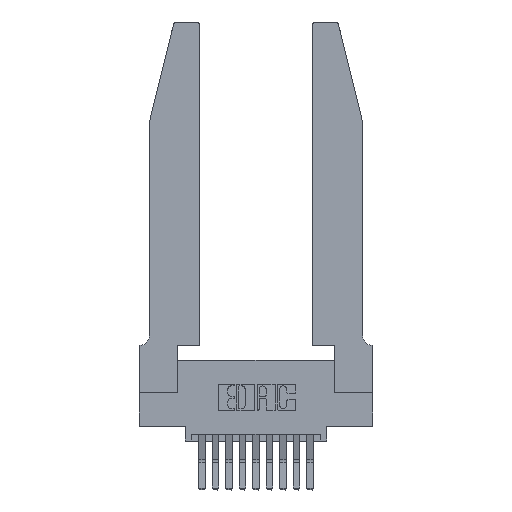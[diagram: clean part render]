
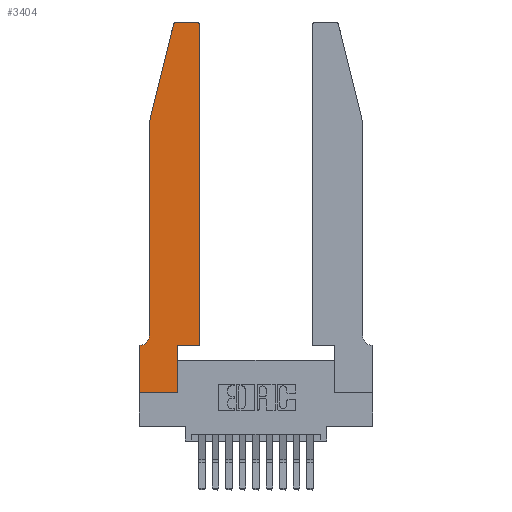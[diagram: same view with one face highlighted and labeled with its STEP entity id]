
A CAD part, top view. The second image highlights one B-rep face of the part: STEP entity #3404.
In plain terms, the highlighted planar face has unit normal (0, 0, 1).
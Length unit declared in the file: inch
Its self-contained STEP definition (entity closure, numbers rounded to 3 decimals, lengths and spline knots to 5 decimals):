
#18 = VERTEX_POINT ( 'NONE', #15408 ) ;
#112 = EDGE_CURVE ( 'NONE', #879, #8846, #6542, .T. ) ;
#124 = DIRECTION ( 'NONE',  ( -1., 0., 0. ) ) ;
#138 = EDGE_CURVE ( 'NONE', #18, #13343, #2961, .T. ) ;
#163 = CARTESIAN_POINT ( 'NONE',  ( 0.284, 2.75, 0.37 ) ) ;
#277 = ORIENTED_EDGE ( 'NONE', *, *, #13344, .T. ) ;
#594 = PLANE ( 'NONE',  #15920 ) ;
#720 = DIRECTION ( 'NONE',  ( 1., 0., 0. ) ) ;
#879 = VERTEX_POINT ( 'NONE', #12487 ) ;
#1127 = CARTESIAN_POINT ( 'NONE',  ( 0., 0., 0.37 ) ) ;
#1167 = VERTEX_POINT ( 'NONE', #163 ) ;
#1363 = CARTESIAN_POINT ( 'NONE',  ( 0.4205, 2.72, 0.37 ) ) ;
#1446 = EDGE_CURVE ( 'NONE', #7575, #16347, #2343, .T. ) ;
#1674 = EDGE_CURVE ( 'NONE', #16347, #2657, #2911, .T. ) ;
#1685 = VECTOR ( 'NONE', #15215, 39.37008 ) ;
#1941 = LINE ( 'NONE', #13389, #10059 ) ;
#2015 = EDGE_CURVE ( 'NONE', #1167, #12087, #8072, .T. ) ;
#2108 = LINE ( 'NONE', #13285, #8444 ) ;
#2284 = EDGE_CURVE ( 'NONE', #16276, #18, #13189, .T. ) ;
#2343 = LINE ( 'NONE', #15055, #3308 ) ;
#2656 = DIRECTION ( 'NONE',  ( 0., 0., 1. ) ) ;
#2657 = VERTEX_POINT ( 'NONE', #7000 ) ;
#2777 = DIRECTION ( 'NONE',  ( 1., 0., 0. ) ) ;
#2823 = FACE_OUTER_BOUND ( 'NONE', #12438, .T. ) ;
#2842 = EDGE_CURVE ( 'NONE', #13343, #1167, #3102, .T. ) ;
#2911 = CIRCLE ( 'NONE', #4374, 0.07 ) ;
#2961 = CIRCLE ( 'NONE', #4784, 0.03 ) ;
#3102 = LINE ( 'NONE', #14027, #4081 ) ;
#3308 = VECTOR ( 'NONE', #16214, 39.37008 ) ;
#3404 = ADVANCED_FACE ( 'NONE', ( #2823 ), #594, .T. ) ;
#4081 = VECTOR ( 'NONE', #6419, 39.37008 ) ;
#4095 = CARTESIAN_POINT ( 'NONE',  ( 0.284, 2.72, 0.37 ) ) ;
#4309 = DIRECTION ( 'NONE',  ( -0.239, -0.971, 0. ) ) ;
#4374 = AXIS2_PLACEMENT_3D ( 'NONE', #15332, #11326, #124 ) ;
#4407 = DIRECTION ( 'NONE',  ( 1., 0., 0. ) ) ;
#4457 = CARTESIAN_POINT ( 'NONE',  ( 0., 0.35, 0.37 ) ) ;
#4784 = AXIS2_PLACEMENT_3D ( 'NONE', #1363, #2656, #12595 ) ;
#5056 = CARTESIAN_POINT ( 'NONE',  ( 0.25487, 2.72718, 0.37 ) ) ;
#5128 = VECTOR ( 'NONE', #7625, 39.37008 ) ;
#5423 = VECTOR ( 'NONE', #2777, 39.37008 ) ;
#5799 = CARTESIAN_POINT ( 'NONE',  ( 0., 0.35, 0.37 ) ) ;
#5970 = EDGE_CURVE ( 'NONE', #2657, #6406, #1941, .T. ) ;
#6122 = ORIENTED_EDGE ( 'NONE', *, *, #2842, .T. ) ;
#6406 = VERTEX_POINT ( 'NONE', #5799 ) ;
#6419 = DIRECTION ( 'NONE',  ( -1., 0., 0. ) ) ;
#6542 = LINE ( 'NONE', #8840, #16332 ) ;
#7000 = CARTESIAN_POINT ( 'NONE',  ( 0.0055, 0.35, 0.37 ) ) ;
#7008 = VECTOR ( 'NONE', #720, 39.37008 ) ;
#7033 = DIRECTION ( 'NONE',  ( -1., 0., 0. ) ) ;
#7223 = EDGE_CURVE ( 'NONE', #12087, #7575, #2108, .T. ) ;
#7575 = VERTEX_POINT ( 'NONE', #13627 ) ;
#7625 = DIRECTION ( 'NONE',  ( 0., -1., 0. ) ) ;
#8072 = CIRCLE ( 'NONE', #9444, 0.03 ) ;
#8258 = VERTEX_POINT ( 'NONE', #1127 ) ;
#8377 = CARTESIAN_POINT ( 'NONE',  ( 0.4505, 0.35, 0.37 ) ) ;
#8444 = VECTOR ( 'NONE', #4309, 39.37008 ) ;
#8840 = CARTESIAN_POINT ( 'NONE',  ( 0.2865, 0.35, 0.37 ) ) ;
#8846 = VERTEX_POINT ( 'NONE', #12315 ) ;
#9150 = LINE ( 'NONE', #13397, #7008 ) ;
#9435 = ORIENTED_EDGE ( 'NONE', *, *, #7223, .T. ) ;
#9444 = AXIS2_PLACEMENT_3D ( 'NONE', #4095, #15449, #12951 ) ;
#10059 = VECTOR ( 'NONE', #7033, 39.37008 ) ;
#10223 = ORIENTED_EDGE ( 'NONE', *, *, #2015, .T. ) ;
#10348 = CARTESIAN_POINT ( 'NONE',  ( 0., 0., 0.37 ) ) ;
#10404 = EDGE_CURVE ( 'NONE', #8258, #879, #10953, .T. ) ;
#10598 = EDGE_CURVE ( 'NONE', #8846, #16276, #9150, .T. ) ;
#10953 = LINE ( 'NONE', #10348, #5423 ) ;
#11326 = DIRECTION ( 'NONE',  ( 0., 0., -1. ) ) ;
#11346 = CARTESIAN_POINT ( 'NONE',  ( 0.4505, 0.35, 0.37 ) ) ;
#11603 = CARTESIAN_POINT ( 'NONE',  ( 0.0755, 0.42, 0.37 ) ) ;
#12035 = LINE ( 'NONE', #15245, #5128 ) ;
#12087 = VERTEX_POINT ( 'NONE', #5056 ) ;
#12315 = CARTESIAN_POINT ( 'NONE',  ( 0.2865, 0.35, 0.37 ) ) ;
#12322 = ORIENTED_EDGE ( 'NONE', *, *, #10598, .T. ) ;
#12438 = EDGE_LOOP ( 'NONE', ( #6122, #10223, #9435, #13163, #14839, #13460, #277, #15935, #13560, #12322, #14319, #16209 ) ) ;
#12487 = CARTESIAN_POINT ( 'NONE',  ( 0.2865, 0., 0.37 ) ) ;
#12595 = DIRECTION ( 'NONE',  ( 1., 0., 0. ) ) ;
#12951 = DIRECTION ( 'NONE',  ( 1., 0., 0. ) ) ;
#13163 = ORIENTED_EDGE ( 'NONE', *, *, #1446, .T. ) ;
#13189 = LINE ( 'NONE', #8377, #1685 ) ;
#13285 = CARTESIAN_POINT ( 'NONE',  ( 0.0755, 2., 0.37 ) ) ;
#13343 = VERTEX_POINT ( 'NONE', #13937 ) ;
#13344 = EDGE_CURVE ( 'NONE', #6406, #8258, #12035, .T. ) ;
#13389 = CARTESIAN_POINT ( 'NONE',  ( 0.0755, 0.35, 0.37 ) ) ;
#13397 = CARTESIAN_POINT ( 'NONE',  ( 0.4505, 0.35, 0.37 ) ) ;
#13460 = ORIENTED_EDGE ( 'NONE', *, *, #5970, .T. ) ;
#13560 = ORIENTED_EDGE ( 'NONE', *, *, #112, .T. ) ;
#13627 = CARTESIAN_POINT ( 'NONE',  ( 0.0755, 2., 0.37 ) ) ;
#13937 = CARTESIAN_POINT ( 'NONE',  ( 0.4205, 2.75, 0.37 ) ) ;
#14027 = CARTESIAN_POINT ( 'NONE',  ( 0.2605, 2.75, 0.37 ) ) ;
#14319 = ORIENTED_EDGE ( 'NONE', *, *, #2284, .T. ) ;
#14839 = ORIENTED_EDGE ( 'NONE', *, *, #1674, .T. ) ;
#15055 = CARTESIAN_POINT ( 'NONE',  ( 0.0755, 2., 0.37 ) ) ;
#15215 = DIRECTION ( 'NONE',  ( 0., 1., 0. ) ) ;
#15245 = CARTESIAN_POINT ( 'NONE',  ( 0., 0., 0.37 ) ) ;
#15261 = DIRECTION ( 'NONE',  ( 0., 1., 0. ) ) ;
#15332 = CARTESIAN_POINT ( 'NONE',  ( 0.0055, 0.42, 0.37 ) ) ;
#15408 = CARTESIAN_POINT ( 'NONE',  ( 0.4505, 2.72, 0.37 ) ) ;
#15449 = DIRECTION ( 'NONE',  ( 0., 0., 1. ) ) ;
#15778 = DIRECTION ( 'NONE',  ( 0., 0., 1. ) ) ;
#15920 = AXIS2_PLACEMENT_3D ( 'NONE', #4457, #15778, #4407 ) ;
#15935 = ORIENTED_EDGE ( 'NONE', *, *, #10404, .T. ) ;
#16209 = ORIENTED_EDGE ( 'NONE', *, *, #138, .T. ) ;
#16214 = DIRECTION ( 'NONE',  ( 0., -1., 0. ) ) ;
#16276 = VERTEX_POINT ( 'NONE', #11346 ) ;
#16332 = VECTOR ( 'NONE', #15261, 39.37008 ) ;
#16347 = VERTEX_POINT ( 'NONE', #11603 ) ;
